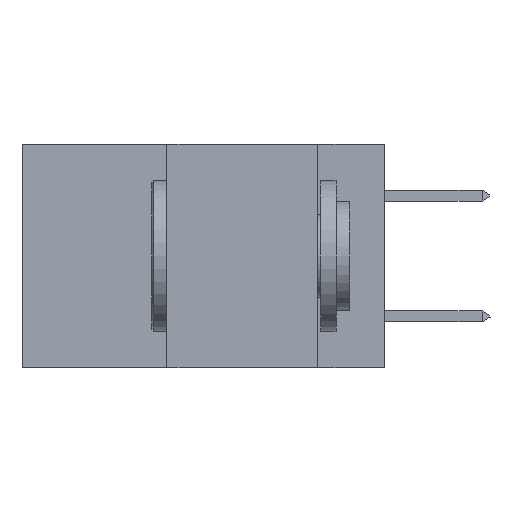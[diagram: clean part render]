
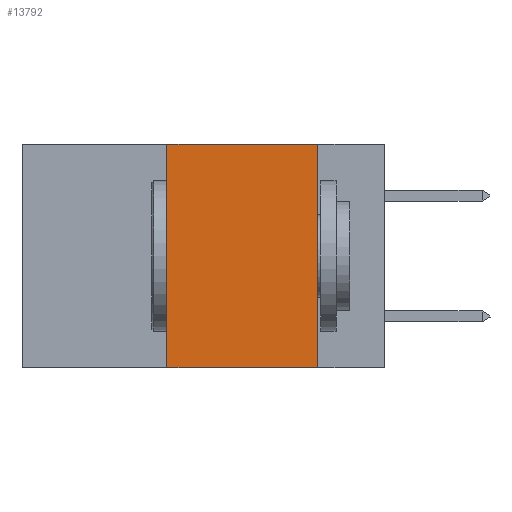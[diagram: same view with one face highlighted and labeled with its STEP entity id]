
A CAD part, left-side view. The second image highlights one B-rep face of the part: STEP entity #13792.
In plain terms, the highlighted planar face has unit normal (-1, 0, 0).
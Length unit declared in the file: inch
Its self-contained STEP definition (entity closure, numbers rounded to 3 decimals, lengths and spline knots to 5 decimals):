
#89 = VERTEX_POINT ( 'NONE', #1793 ) ;
#1043 = DIRECTION ( 'NONE',  ( 0., 0., -1. ) ) ;
#1065 = ORIENTED_EDGE ( 'NONE', *, *, #12269, .F. ) ;
#1516 = VERTEX_POINT ( 'NONE', #3074 ) ;
#1756 = LINE ( 'NONE', #13561, #4702 ) ;
#1793 = CARTESIAN_POINT ( 'NONE',  ( 0., 0.11, -0.37 ) ) ;
#2311 = EDGE_CURVE ( 'NONE', #3025, #1516, #12096, .T. ) ;
#2750 = VERTEX_POINT ( 'NONE', #3267 ) ;
#3025 = VERTEX_POINT ( 'NONE', #13877 ) ;
#3074 = CARTESIAN_POINT ( 'NONE',  ( 0., 0.36, 0. ) ) ;
#3267 = CARTESIAN_POINT ( 'NONE',  ( 0., 0.11, 0. ) ) ;
#3640 = FACE_OUTER_BOUND ( 'NONE', #8870, .T. ) ;
#4025 = DIRECTION ( 'NONE',  ( 0., -1., 0. ) ) ;
#4509 = CARTESIAN_POINT ( 'NONE',  ( 0., 0.6, 0. ) ) ;
#4702 = VECTOR ( 'NONE', #14820, 39.37008 ) ;
#4999 = CARTESIAN_POINT ( 'NONE',  ( 0., 0.36, 0. ) ) ;
#5853 = LINE ( 'NONE', #12869, #12168 ) ;
#7011 = PLANE ( 'NONE',  #10447 ) ;
#7053 = LINE ( 'NONE', #8569, #7835 ) ;
#7835 = VECTOR ( 'NONE', #1043, 39.37008 ) ;
#7909 = ORIENTED_EDGE ( 'NONE', *, *, #2311, .F. ) ;
#8329 = DIRECTION ( 'NONE',  ( 0., 0., -1. ) ) ;
#8569 = CARTESIAN_POINT ( 'NONE',  ( 0., 0.11, 0. ) ) ;
#8870 = EDGE_LOOP ( 'NONE', ( #9961, #1065, #7909, #14488 ) ) ;
#9961 = ORIENTED_EDGE ( 'NONE', *, *, #10763, .F. ) ;
#10020 = EDGE_CURVE ( 'NONE', #3025, #89, #1756, .T. ) ;
#10088 = DIRECTION ( 'NONE',  ( 0., 0., 1. ) ) ;
#10447 = AXIS2_PLACEMENT_3D ( 'NONE', #4509, #15856, #8329 ) ;
#10763 = EDGE_CURVE ( 'NONE', #2750, #89, #7053, .T. ) ;
#11710 = VECTOR ( 'NONE', #10088, 39.37008 ) ;
#12096 = LINE ( 'NONE', #4999, #11710 ) ;
#12168 = VECTOR ( 'NONE', #4025, 39.37008 ) ;
#12269 = EDGE_CURVE ( 'NONE', #1516, #2750, #5853, .T. ) ;
#12869 = CARTESIAN_POINT ( 'NONE',  ( 0., 0.6, 0. ) ) ;
#13561 = CARTESIAN_POINT ( 'NONE',  ( 0., 0.6, -0.37 ) ) ;
#13792 = ADVANCED_FACE ( 'NONE', ( #3640 ), #7011, .F. ) ;
#13877 = CARTESIAN_POINT ( 'NONE',  ( 0., 0.36, -0.37 ) ) ;
#14488 = ORIENTED_EDGE ( 'NONE', *, *, #10020, .T. ) ;
#14820 = DIRECTION ( 'NONE',  ( 0., -1., 0. ) ) ;
#15856 = DIRECTION ( 'NONE',  ( 1., 0., 0. ) ) ;
